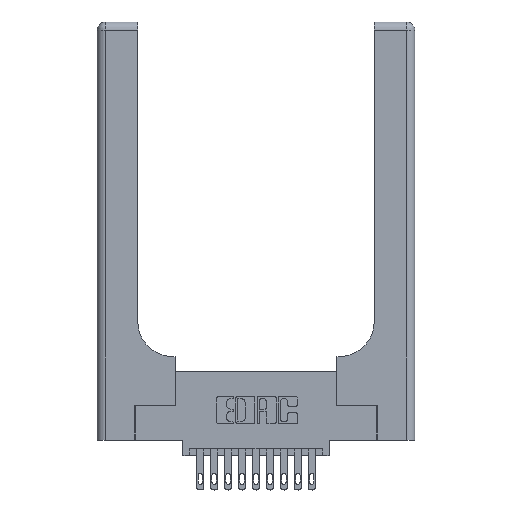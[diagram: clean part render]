
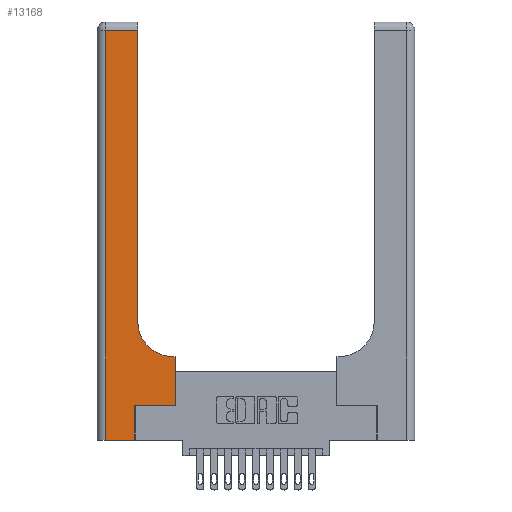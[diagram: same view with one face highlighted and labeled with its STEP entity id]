
A CAD part, top view. The second image highlights one B-rep face of the part: STEP entity #13168.
In plain terms, the highlighted planar face has unit normal (0, 0, 1).
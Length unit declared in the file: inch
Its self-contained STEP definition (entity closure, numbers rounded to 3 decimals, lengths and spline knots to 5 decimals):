
#230 = CARTESIAN_POINT ( 'NONE',  ( 0.5585, 0.25, 0.37 ) ) ;
#797 = EDGE_CURVE ( 'NONE', #14272, #11608, #3328, .T. ) ;
#838 = CARTESIAN_POINT ( 'NONE',  ( 0.269, 0.25, 0.37 ) ) ;
#947 = EDGE_CURVE ( 'NONE', #7798, #1211, #9791, .T. ) ;
#1187 = EDGE_CURVE ( 'NONE', #5613, #15682, #6945, .T. ) ;
#1211 = VERTEX_POINT ( 'NONE', #2012 ) ;
#1402 = EDGE_CURVE ( 'NONE', #16709, #14302, #6122, .T. ) ;
#1693 = CIRCLE ( 'NONE', #9357, 0.25 ) ;
#1934 = ORIENTED_EDGE ( 'NONE', *, *, #8361, .T. ) ;
#1954 = CARTESIAN_POINT ( 'NONE',  ( 0.5415, 0.6, 0.37 ) ) ;
#2012 = CARTESIAN_POINT ( 'NONE',  ( 0.2915, 2.94, 0.37 ) ) ;
#2113 = DIRECTION ( 'NONE',  ( -1., 0., 0. ) ) ;
#2119 = CARTESIAN_POINT ( 'NONE',  ( 0.2915, 0.85, 0.37 ) ) ;
#2255 = CARTESIAN_POINT ( 'NONE',  ( 0.2915, 0.6, 0.37 ) ) ;
#2361 = FACE_OUTER_BOUND ( 'NONE', #5017, .T. ) ;
#2924 = VECTOR ( 'NONE', #3966, 39.37008 ) ;
#2999 = ORIENTED_EDGE ( 'NONE', *, *, #11389, .T. ) ;
#3159 = VERTEX_POINT ( 'NONE', #15955 ) ;
#3328 = LINE ( 'NONE', #7140, #13586 ) ;
#3430 = DIRECTION ( 'NONE',  ( 1., 0., 0. ) ) ;
#3570 = DIRECTION ( 'NONE',  ( 1., 0., 0. ) ) ;
#3724 = VECTOR ( 'NONE', #5094, 39.37008 ) ;
#3966 = DIRECTION ( 'NONE',  ( 0., 1., 0. ) ) ;
#4256 = LINE ( 'NONE', #8279, #8519 ) ;
#4473 = CARTESIAN_POINT ( 'NONE',  ( 0.269, 0., 0.37 ) ) ;
#4527 = LINE ( 'NONE', #9188, #14008 ) ;
#5017 = EDGE_LOOP ( 'NONE', ( #7112, #1934, #15720, #14706, #2999, #13974, #10992, #13276, #9803 ) ) ;
#5094 = DIRECTION ( 'NONE',  ( -1., 0., 0. ) ) ;
#5613 = VERTEX_POINT ( 'NONE', #5949 ) ;
#5904 = VECTOR ( 'NONE', #3430, 39.37008 ) ;
#5938 = DIRECTION ( 'NONE',  ( 0., -1., 0. ) ) ;
#5949 = CARTESIAN_POINT ( 'NONE',  ( 0.269, 0.25, 0.37 ) ) ;
#6122 = LINE ( 'NONE', #2255, #3724 ) ;
#6203 = CARTESIAN_POINT ( 'NONE',  ( 0.5585, 0.6, 0.37 ) ) ;
#6945 = LINE ( 'NONE', #838, #5904 ) ;
#7067 = DIRECTION ( 'NONE',  ( 0., 1., 0. ) ) ;
#7112 = ORIENTED_EDGE ( 'NONE', *, *, #947, .T. ) ;
#7140 = CARTESIAN_POINT ( 'NONE',  ( 0.06, 3., 0.37 ) ) ;
#7798 = VERTEX_POINT ( 'NONE', #2119 ) ;
#7879 = DIRECTION ( 'NONE',  ( 1., 0., 0. ) ) ;
#8219 = DIRECTION ( 'NONE',  ( -1., 0., 0. ) ) ;
#8279 = CARTESIAN_POINT ( 'NONE',  ( 0.5585, 0.25, 0.37 ) ) ;
#8361 = EDGE_CURVE ( 'NONE', #1211, #14272, #12185, .T. ) ;
#8519 = VECTOR ( 'NONE', #14462, 39.37008 ) ;
#8641 = CARTESIAN_POINT ( 'NONE',  ( 0., 3., 0.37 ) ) ;
#8794 = AXIS2_PLACEMENT_3D ( 'NONE', #8641, #15119, #2113 ) ;
#8795 = VECTOR ( 'NONE', #8219, 39.37008 ) ;
#9188 = CARTESIAN_POINT ( 'NONE',  ( 0., 0., 0.37 ) ) ;
#9357 = AXIS2_PLACEMENT_3D ( 'NONE', #13739, #15211, #3570 ) ;
#9791 = LINE ( 'NONE', #10675, #2924 ) ;
#9803 = ORIENTED_EDGE ( 'NONE', *, *, #15380, .T. ) ;
#9959 = CARTESIAN_POINT ( 'NONE',  ( 0.06, 0., 0.37 ) ) ;
#10477 = EDGE_CURVE ( 'NONE', #15682, #16709, #4256, .T. ) ;
#10675 = CARTESIAN_POINT ( 'NONE',  ( 0.2915, 3., 0.37 ) ) ;
#10992 = ORIENTED_EDGE ( 'NONE', *, *, #10477, .T. ) ;
#11389 = EDGE_CURVE ( 'NONE', #3159, #5613, #15958, .T. ) ;
#11608 = VERTEX_POINT ( 'NONE', #9959 ) ;
#12185 = LINE ( 'NONE', #14741, #8795 ) ;
#13168 = ADVANCED_FACE ( 'NONE', ( #2361 ), #16253, .F. ) ;
#13276 = ORIENTED_EDGE ( 'NONE', *, *, #1402, .T. ) ;
#13586 = VECTOR ( 'NONE', #5938, 39.37008 ) ;
#13739 = CARTESIAN_POINT ( 'NONE',  ( 0.5415, 0.85, 0.37 ) ) ;
#13974 = ORIENTED_EDGE ( 'NONE', *, *, #1187, .T. ) ;
#14008 = VECTOR ( 'NONE', #7879, 39.37008 ) ;
#14272 = VERTEX_POINT ( 'NONE', #16215 ) ;
#14302 = VERTEX_POINT ( 'NONE', #1954 ) ;
#14462 = DIRECTION ( 'NONE',  ( 0., 1., 0. ) ) ;
#14706 = ORIENTED_EDGE ( 'NONE', *, *, #15006, .T. ) ;
#14741 = CARTESIAN_POINT ( 'NONE',  ( 0., 2.94, 0.37 ) ) ;
#14904 = VECTOR ( 'NONE', #7067, 39.37008 ) ;
#15006 = EDGE_CURVE ( 'NONE', #11608, #3159, #4527, .T. ) ;
#15119 = DIRECTION ( 'NONE',  ( 0., 0., -1. ) ) ;
#15211 = DIRECTION ( 'NONE',  ( 0., 0., -1. ) ) ;
#15380 = EDGE_CURVE ( 'NONE', #14302, #7798, #1693, .T. ) ;
#15682 = VERTEX_POINT ( 'NONE', #230 ) ;
#15720 = ORIENTED_EDGE ( 'NONE', *, *, #797, .T. ) ;
#15955 = CARTESIAN_POINT ( 'NONE',  ( 0.269, 0., 0.37 ) ) ;
#15958 = LINE ( 'NONE', #4473, #14904 ) ;
#16215 = CARTESIAN_POINT ( 'NONE',  ( 0.06, 2.94, 0.37 ) ) ;
#16253 = PLANE ( 'NONE',  #8794 ) ;
#16709 = VERTEX_POINT ( 'NONE', #6203 ) ;
